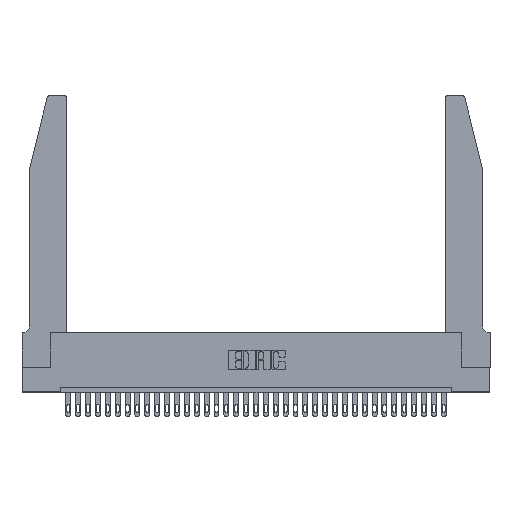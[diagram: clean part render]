
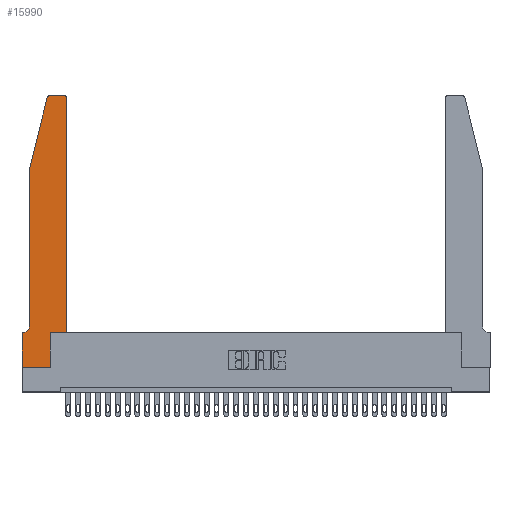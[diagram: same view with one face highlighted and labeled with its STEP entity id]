
A CAD part, top view. The second image highlights one B-rep face of the part: STEP entity #15990.
In plain terms, the highlighted planar face has unit normal (0, 0, 1).
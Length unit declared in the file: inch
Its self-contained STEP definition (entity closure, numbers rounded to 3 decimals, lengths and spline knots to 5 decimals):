
#862 = CARTESIAN_POINT ( 'NONE',  ( 0.284, 2.72, 0.37 ) ) ;
#900 = CIRCLE ( 'NONE', #10587, 0.07 ) ;
#1412 = CARTESIAN_POINT ( 'NONE',  ( 0., 0., 0.37 ) ) ;
#1467 = CARTESIAN_POINT ( 'NONE',  ( 0.4505, 0.35, 0.37 ) ) ;
#2102 = EDGE_CURVE ( 'NONE', #28292, #17109, #25249, .T. ) ;
#2913 = LINE ( 'NONE', #32283, #21992 ) ;
#3206 = ORIENTED_EDGE ( 'NONE', *, *, #25586, .T. ) ;
#3237 = CIRCLE ( 'NONE', #9433, 0.03 ) ;
#3739 = CARTESIAN_POINT ( 'NONE',  ( 0.0055, 0.35, 0.37 ) ) ;
#3926 = EDGE_CURVE ( 'NONE', #29146, #10483, #33874, .T. ) ;
#4124 = CARTESIAN_POINT ( 'NONE',  ( 0.4505, 2.72, 0.37 ) ) ;
#4231 = LINE ( 'NONE', #33462, #5452 ) ;
#4531 = CARTESIAN_POINT ( 'NONE',  ( 0., 0.35, 0.37 ) ) ;
#4979 = DIRECTION ( 'NONE',  ( 0., 0., 1. ) ) ;
#5452 = VECTOR ( 'NONE', #14370, 39.37008 ) ;
#5814 = DIRECTION ( 'NONE',  ( 0., 0., 1. ) ) ;
#5943 = ORIENTED_EDGE ( 'NONE', *, *, #18279, .T. ) ;
#6032 = EDGE_LOOP ( 'NONE', ( #8253, #29605, #25615, #3206, #5943, #15189, #28244, #14269, #18824, #10397, #31420, #14540 ) ) ;
#6147 = LINE ( 'NONE', #9947, #26996 ) ;
#6170 = CARTESIAN_POINT ( 'NONE',  ( 0.4205, 2.75, 0.37 ) ) ;
#6356 = CARTESIAN_POINT ( 'NONE',  ( 0.2865, 0., 0.37 ) ) ;
#6393 = CARTESIAN_POINT ( 'NONE',  ( 0.2865, 0.35, 0.37 ) ) ;
#6495 = CIRCLE ( 'NONE', #19115, 0.03 ) ;
#6517 = VECTOR ( 'NONE', #14150, 39.37008 ) ;
#6622 = VERTEX_POINT ( 'NONE', #17948 ) ;
#6679 = EDGE_CURVE ( 'NONE', #13397, #16280, #4231, .T. ) ;
#6795 = DIRECTION ( 'NONE',  ( 0., 1., 0. ) ) ;
#7358 = CARTESIAN_POINT ( 'NONE',  ( 0.0055, 0.42, 0.37 ) ) ;
#7789 = CARTESIAN_POINT ( 'NONE',  ( 0.0755, 0.42, 0.37 ) ) ;
#7885 = DIRECTION ( 'NONE',  ( 1., 0., 0. ) ) ;
#7960 = EDGE_CURVE ( 'NONE', #6622, #17534, #3237, .T. ) ;
#8052 = EDGE_CURVE ( 'NONE', #12258, #6622, #6147, .T. ) ;
#8146 = CARTESIAN_POINT ( 'NONE',  ( 0.0755, 0.35, 0.37 ) ) ;
#8246 = DIRECTION ( 'NONE',  ( -1., 0., 0. ) ) ;
#8253 = ORIENTED_EDGE ( 'NONE', *, *, #8052, .T. ) ;
#8581 = FACE_OUTER_BOUND ( 'NONE', #6032, .T. ) ;
#9433 = AXIS2_PLACEMENT_3D ( 'NONE', #862, #5814, #26943 ) ;
#9947 = CARTESIAN_POINT ( 'NONE',  ( 0.2605, 2.75, 0.37 ) ) ;
#10397 = ORIENTED_EDGE ( 'NONE', *, *, #22062, .T. ) ;
#10483 = VERTEX_POINT ( 'NONE', #28767 ) ;
#10587 = AXIS2_PLACEMENT_3D ( 'NONE', #7358, #12706, #20686 ) ;
#11044 = DIRECTION ( 'NONE',  ( 1., 0., 0. ) ) ;
#11334 = LINE ( 'NONE', #26610, #20734 ) ;
#12258 = VERTEX_POINT ( 'NONE', #6170 ) ;
#12706 = DIRECTION ( 'NONE',  ( 0., 0., -1. ) ) ;
#12716 = VERTEX_POINT ( 'NONE', #1412 ) ;
#13397 = VERTEX_POINT ( 'NONE', #6356 ) ;
#13882 = VECTOR ( 'NONE', #18226, 39.37008 ) ;
#14150 = DIRECTION ( 'NONE',  ( 0., -1., 0. ) ) ;
#14269 = ORIENTED_EDGE ( 'NONE', *, *, #34028, .T. ) ;
#14370 = DIRECTION ( 'NONE',  ( 0., 1., 0. ) ) ;
#14540 = ORIENTED_EDGE ( 'NONE', *, *, #31092, .T. ) ;
#15189 = ORIENTED_EDGE ( 'NONE', *, *, #3926, .T. ) ;
#15561 = CARTESIAN_POINT ( 'NONE',  ( 0.4505, 0.35, 0.37 ) ) ;
#15990 = ADVANCED_FACE ( 'NONE', ( #8581 ), #20427, .T. ) ;
#16030 = DIRECTION ( 'NONE',  ( -0.239, -0.971, 0. ) ) ;
#16280 = VERTEX_POINT ( 'NONE', #6393 ) ;
#17109 = VERTEX_POINT ( 'NONE', #4124 ) ;
#17211 = LINE ( 'NONE', #15561, #13882 ) ;
#17534 = VERTEX_POINT ( 'NONE', #25356 ) ;
#17718 = VECTOR ( 'NONE', #28070, 39.37008 ) ;
#17948 = CARTESIAN_POINT ( 'NONE',  ( 0.284, 2.75, 0.37 ) ) ;
#18205 = CARTESIAN_POINT ( 'NONE',  ( 0.4205, 2.72, 0.37 ) ) ;
#18226 = DIRECTION ( 'NONE',  ( 1., 0., 0. ) ) ;
#18279 = EDGE_CURVE ( 'NONE', #28241, #29146, #900, .T. ) ;
#18824 = ORIENTED_EDGE ( 'NONE', *, *, #6679, .T. ) ;
#19115 = AXIS2_PLACEMENT_3D ( 'NONE', #18205, #4979, #23508 ) ;
#19904 = EDGE_CURVE ( 'NONE', #17534, #28225, #11334, .T. ) ;
#20427 = PLANE ( 'NONE',  #24047 ) ;
#20686 = DIRECTION ( 'NONE',  ( -1., 0., 0. ) ) ;
#20734 = VECTOR ( 'NONE', #16030, 39.37008 ) ;
#21430 = LINE ( 'NONE', #25161, #6517 ) ;
#21992 = VECTOR ( 'NONE', #11044, 39.37008 ) ;
#22062 = EDGE_CURVE ( 'NONE', #16280, #28292, #17211, .T. ) ;
#22729 = VECTOR ( 'NONE', #6795, 39.37008 ) ;
#22930 = CARTESIAN_POINT ( 'NONE',  ( 0., 0., 0.37 ) ) ;
#23508 = DIRECTION ( 'NONE',  ( 1., 0., 0. ) ) ;
#24047 = AXIS2_PLACEMENT_3D ( 'NONE', #4531, #25756, #7885 ) ;
#25161 = CARTESIAN_POINT ( 'NONE',  ( 0.0755, 2., 0.37 ) ) ;
#25249 = LINE ( 'NONE', #1467, #22729 ) ;
#25356 = CARTESIAN_POINT ( 'NONE',  ( 0.25487, 2.72718, 0.37 ) ) ;
#25586 = EDGE_CURVE ( 'NONE', #28225, #28241, #21430, .T. ) ;
#25615 = ORIENTED_EDGE ( 'NONE', *, *, #19904, .T. ) ;
#25742 = EDGE_CURVE ( 'NONE', #10483, #12716, #29316, .T. ) ;
#25756 = DIRECTION ( 'NONE',  ( 0., 0., 1. ) ) ;
#26610 = CARTESIAN_POINT ( 'NONE',  ( 0.0755, 2., 0.37 ) ) ;
#26943 = DIRECTION ( 'NONE',  ( 1., 0., 0. ) ) ;
#26996 = VECTOR ( 'NONE', #31284, 39.37008 ) ;
#28070 = DIRECTION ( 'NONE',  ( 0., -1., 0. ) ) ;
#28225 = VERTEX_POINT ( 'NONE', #29880 ) ;
#28241 = VERTEX_POINT ( 'NONE', #7789 ) ;
#28244 = ORIENTED_EDGE ( 'NONE', *, *, #25742, .T. ) ;
#28292 = VERTEX_POINT ( 'NONE', #32455 ) ;
#28767 = CARTESIAN_POINT ( 'NONE',  ( 0., 0.35, 0.37 ) ) ;
#29146 = VERTEX_POINT ( 'NONE', #3739 ) ;
#29316 = LINE ( 'NONE', #22930, #17718 ) ;
#29605 = ORIENTED_EDGE ( 'NONE', *, *, #7960, .T. ) ;
#29880 = CARTESIAN_POINT ( 'NONE',  ( 0.0755, 2., 0.37 ) ) ;
#30053 = VECTOR ( 'NONE', #8246, 39.37008 ) ;
#31092 = EDGE_CURVE ( 'NONE', #17109, #12258, #6495, .T. ) ;
#31284 = DIRECTION ( 'NONE',  ( -1., 0., 0. ) ) ;
#31420 = ORIENTED_EDGE ( 'NONE', *, *, #2102, .T. ) ;
#32283 = CARTESIAN_POINT ( 'NONE',  ( 0., 0., 0.37 ) ) ;
#32455 = CARTESIAN_POINT ( 'NONE',  ( 0.4505, 0.35, 0.37 ) ) ;
#33462 = CARTESIAN_POINT ( 'NONE',  ( 0.2865, 0.35, 0.37 ) ) ;
#33874 = LINE ( 'NONE', #8146, #30053 ) ;
#34028 = EDGE_CURVE ( 'NONE', #12716, #13397, #2913, .T. ) ;
